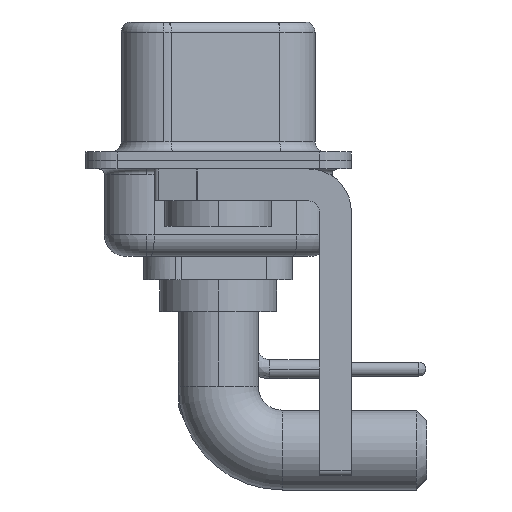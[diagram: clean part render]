
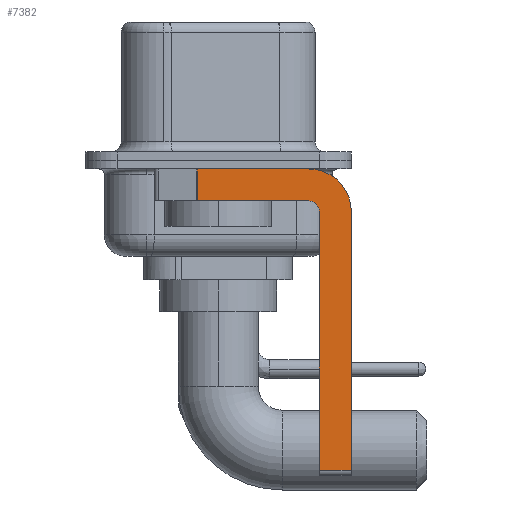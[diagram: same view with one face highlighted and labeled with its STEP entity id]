
A CAD part, left-side view. The second image highlights one B-rep face of the part: STEP entity #7382.
In plain terms, the highlighted planar face has unit normal (-1, 0, 0).
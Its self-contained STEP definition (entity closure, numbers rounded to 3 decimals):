
#299 = FACE_OUTER_BOUND ( 'NONE', #12205, .T. ) ;
#1005 = ORIENTED_EDGE ( 'NONE', *, *, #14774, .T. ) ;
#1400 = CARTESIAN_POINT ( 'NONE',  ( -2.9, 0.978, -1.9 ) ) ;
#1609 = CARTESIAN_POINT ( 'NONE',  ( -2.9, -4.75, -14.8 ) ) ;
#1614 = DIRECTION ( 'NONE',  ( 0., -1., 0. ) ) ;
#1975 = DIRECTION ( 'NONE',  ( 0., 0., -1. ) ) ;
#2056 = ORIENTED_EDGE ( 'NONE', *, *, #9242, .F. ) ;
#2684 = CARTESIAN_POINT ( 'NONE',  ( -2.9, -4.25, -0.4 ) ) ;
#3562 = CARTESIAN_POINT ( 'NONE',  ( -2.9, 0.978, -0.4 ) ) ;
#3797 = CARTESIAN_POINT ( 'NONE',  ( -2.9, -6.25, -2.4 ) ) ;
#4136 = CARTESIAN_POINT ( 'NONE',  ( -2.9, -4.75, -2.4 ) ) ;
#4676 = VERTEX_POINT ( 'NONE', #16450 ) ;
#5025 = DIRECTION ( 'NONE',  ( 0., 0., -1. ) ) ;
#5075 = VECTOR ( 'NONE', #23857, 1000. ) ;
#5654 = CARTESIAN_POINT ( 'NONE',  ( -2.9, -4.25, -14.55 ) ) ;
#6047 = LINE ( 'NONE', #5654, #24990 ) ;
#7382 = ADVANCED_FACE ( 'NONE', ( #299 ), #17114, .F. ) ;
#7387 = VECTOR ( 'NONE', #18413, 1000. ) ;
#7459 = LINE ( 'NONE', #7590, #5075 ) ;
#7590 = CARTESIAN_POINT ( 'NONE',  ( -2.9, -4.25, -1.9 ) ) ;
#8187 = VERTEX_POINT ( 'NONE', #10727 ) ;
#8341 = DIRECTION ( 'NONE',  ( 0., 0., 1. ) ) ;
#9242 = EDGE_CURVE ( 'NONE', #25649, #11046, #9762, .T. ) ;
#9333 = VECTOR ( 'NONE', #26573, 1000. ) ;
#9716 = EDGE_CURVE ( 'NONE', #15098, #25649, #10624, .T. ) ;
#9762 = LINE ( 'NONE', #16227, #18361 ) ;
#9782 = AXIS2_PLACEMENT_3D ( 'NONE', #26395, #14186, #16068 ) ;
#9846 = EDGE_CURVE ( 'NONE', #8187, #4676, #7459, .T. ) ;
#10142 = ORIENTED_EDGE ( 'NONE', *, *, #16974, .T. ) ;
#10175 = LINE ( 'NONE', #1609, #7387 ) ;
#10624 = CIRCLE ( 'NONE', #9782, 2. ) ;
#10727 = CARTESIAN_POINT ( 'NONE',  ( -2.9, -4.25, -1.9 ) ) ;
#11046 = VERTEX_POINT ( 'NONE', #18349 ) ;
#12091 = CARTESIAN_POINT ( 'NONE',  ( -2.9, -4.75, -14.55 ) ) ;
#12205 = EDGE_LOOP ( 'NONE', ( #14703, #1005, #15492, #14365, #19528, #10142, #2056, #21956 ) ) ;
#12224 = CARTESIAN_POINT ( 'NONE',  ( -2.9, -4.25, -2.4 ) ) ;
#13121 = AXIS2_PLACEMENT_3D ( 'NONE', #16718, #24919, #18878 ) ;
#13280 = VERTEX_POINT ( 'NONE', #12091 ) ;
#13738 = VERTEX_POINT ( 'NONE', #4136 ) ;
#14186 = DIRECTION ( 'NONE',  ( 1., 0., 0. ) ) ;
#14365 = ORIENTED_EDGE ( 'NONE', *, *, #18261, .F. ) ;
#14703 = ORIENTED_EDGE ( 'NONE', *, *, #17311, .F. ) ;
#14774 = EDGE_CURVE ( 'NONE', #23920, #4676, #17405, .T. ) ;
#15098 = VERTEX_POINT ( 'NONE', #2684 ) ;
#15492 = ORIENTED_EDGE ( 'NONE', *, *, #9846, .F. ) ;
#15561 = EDGE_CURVE ( 'NONE', #13280, #13738, #10175, .T. ) ;
#16068 = DIRECTION ( 'NONE',  ( 0., 0., -1. ) ) ;
#16102 = CARTESIAN_POINT ( 'NONE',  ( -2.9, 3., -0.4 ) ) ;
#16227 = CARTESIAN_POINT ( 'NONE',  ( -2.9, -6.25, -2.4 ) ) ;
#16450 = CARTESIAN_POINT ( 'NONE',  ( -2.9, 0.978, -1.9 ) ) ;
#16718 = CARTESIAN_POINT ( 'NONE',  ( -2.9, -4.25, -2.4 ) ) ;
#16974 = EDGE_CURVE ( 'NONE', #13280, #11046, #6047, .T. ) ;
#17114 = PLANE ( 'NONE',  #13121 ) ;
#17311 = EDGE_CURVE ( 'NONE', #23920, #15098, #26432, .T. ) ;
#17405 = LINE ( 'NONE', #1400, #21518 ) ;
#18261 = EDGE_CURVE ( 'NONE', #13738, #8187, #25268, .T. ) ;
#18349 = CARTESIAN_POINT ( 'NONE',  ( -2.9, -6.25, -14.55 ) ) ;
#18361 = VECTOR ( 'NONE', #1975, 1000. ) ;
#18413 = DIRECTION ( 'NONE',  ( 0., 0., 1. ) ) ;
#18878 = DIRECTION ( 'NONE',  ( 0., 0., -1. ) ) ;
#19528 = ORIENTED_EDGE ( 'NONE', *, *, #15561, .F. ) ;
#21518 = VECTOR ( 'NONE', #5025, 1000. ) ;
#21956 = ORIENTED_EDGE ( 'NONE', *, *, #9716, .F. ) ;
#22166 = DIRECTION ( 'NONE',  ( -1., 0., 0. ) ) ;
#23118 = AXIS2_PLACEMENT_3D ( 'NONE', #12224, #22166, #8341 ) ;
#23857 = DIRECTION ( 'NONE',  ( 0., 1., 0. ) ) ;
#23920 = VERTEX_POINT ( 'NONE', #3562 ) ;
#24919 = DIRECTION ( 'NONE',  ( 1., 0., 0. ) ) ;
#24990 = VECTOR ( 'NONE', #1614, 1000. ) ;
#25268 = CIRCLE ( 'NONE', #23118, 0.5 ) ;
#25649 = VERTEX_POINT ( 'NONE', #3797 ) ;
#26395 = CARTESIAN_POINT ( 'NONE',  ( -2.9, -4.25, -2.4 ) ) ;
#26432 = LINE ( 'NONE', #16102, #9333 ) ;
#26573 = DIRECTION ( 'NONE',  ( 0., -1., 0. ) ) ;
